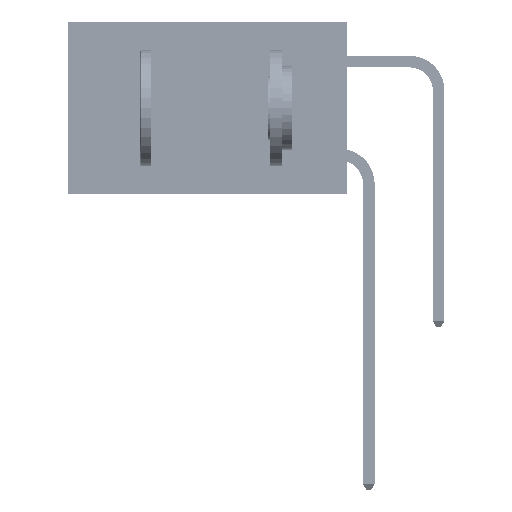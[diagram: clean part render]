
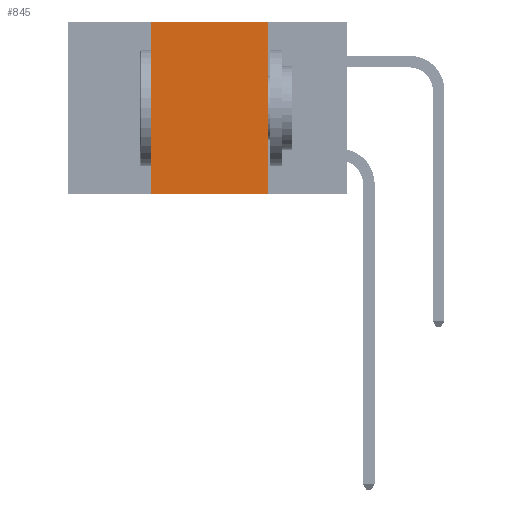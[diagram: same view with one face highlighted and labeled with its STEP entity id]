
A CAD part, left-side view. The second image highlights one B-rep face of the part: STEP entity #845.
In plain terms, the highlighted planar face has unit normal (-1, 0, 0).
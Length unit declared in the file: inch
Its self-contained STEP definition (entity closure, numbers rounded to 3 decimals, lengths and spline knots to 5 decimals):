
#632 = CARTESIAN_POINT ( 'NONE',  ( 0., 0.6, -0.37 ) ) ;
#845 = ADVANCED_FACE ( 'NONE', ( #43211 ), #47111, .F. ) ;
#1539 = ORIENTED_EDGE ( 'NONE', *, *, #48048, .F. ) ;
#1942 = ORIENTED_EDGE ( 'NONE', *, *, #32455, .F. ) ;
#3274 = VERTEX_POINT ( 'NONE', #33859 ) ;
#3624 = EDGE_LOOP ( 'NONE', ( #1539, #7899, #1942, #20960 ) ) ;
#4322 = DIRECTION ( 'NONE',  ( 0., 0., -1. ) ) ;
#7899 = ORIENTED_EDGE ( 'NONE', *, *, #19254, .F. ) ;
#10209 = VERTEX_POINT ( 'NONE', #35407 ) ;
#12084 = CARTESIAN_POINT ( 'NONE',  ( 0., 0.42, 0. ) ) ;
#19254 = EDGE_CURVE ( 'NONE', #3274, #40815, #24059, .T. ) ;
#20123 = EDGE_CURVE ( 'NONE', #10209, #47274, #35105, .T. ) ;
#20507 = VECTOR ( 'NONE', #41345, 39.37008 ) ;
#20889 = AXIS2_PLACEMENT_3D ( 'NONE', #21864, #25581, #4322 ) ;
#20960 = ORIENTED_EDGE ( 'NONE', *, *, #20123, .T. ) ;
#21864 = CARTESIAN_POINT ( 'NONE',  ( 0., 0.6, 0. ) ) ;
#23928 = CARTESIAN_POINT ( 'NONE',  ( 0., 0.17, -0.37 ) ) ;
#24059 = LINE ( 'NONE', #28706, #33972 ) ;
#25581 = DIRECTION ( 'NONE',  ( 1., 0., 0. ) ) ;
#28706 = CARTESIAN_POINT ( 'NONE',  ( 0., 0.6, 0. ) ) ;
#28877 = DIRECTION ( 'NONE',  ( 0., -1., 0. ) ) ;
#32147 = VECTOR ( 'NONE', #43102, 39.37008 ) ;
#32455 = EDGE_CURVE ( 'NONE', #10209, #3274, #39031, .T. ) ;
#33805 = VECTOR ( 'NONE', #34935, 39.37008 ) ;
#33859 = CARTESIAN_POINT ( 'NONE',  ( 0., 0.42, 0. ) ) ;
#33972 = VECTOR ( 'NONE', #28877, 39.37008 ) ;
#34935 = DIRECTION ( 'NONE',  ( 0., 0., 1. ) ) ;
#35105 = LINE ( 'NONE', #632, #20507 ) ;
#35407 = CARTESIAN_POINT ( 'NONE',  ( 0., 0.42, -0.37 ) ) ;
#38243 = CARTESIAN_POINT ( 'NONE',  ( 0., 0.17, 0. ) ) ;
#38690 = CARTESIAN_POINT ( 'NONE',  ( 0., 0.17, 0. ) ) ;
#39031 = LINE ( 'NONE', #12084, #33805 ) ;
#40815 = VERTEX_POINT ( 'NONE', #38243 ) ;
#41345 = DIRECTION ( 'NONE',  ( 0., -1., 0. ) ) ;
#43102 = DIRECTION ( 'NONE',  ( 0., 0., -1. ) ) ;
#43211 = FACE_OUTER_BOUND ( 'NONE', #3624, .T. ) ;
#44923 = LINE ( 'NONE', #38690, #32147 ) ;
#47111 = PLANE ( 'NONE',  #20889 ) ;
#47274 = VERTEX_POINT ( 'NONE', #23928 ) ;
#48048 = EDGE_CURVE ( 'NONE', #40815, #47274, #44923, .T. ) ;
